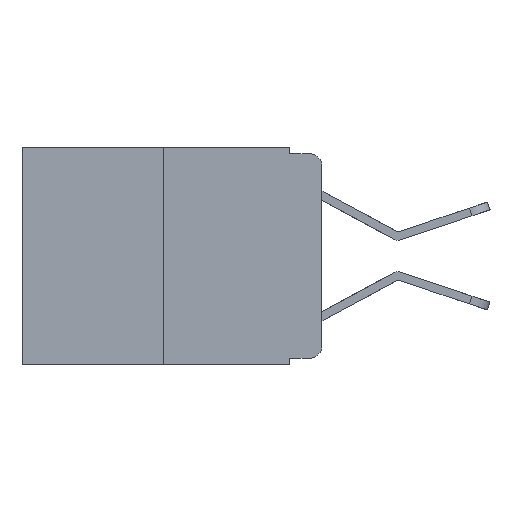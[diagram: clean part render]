
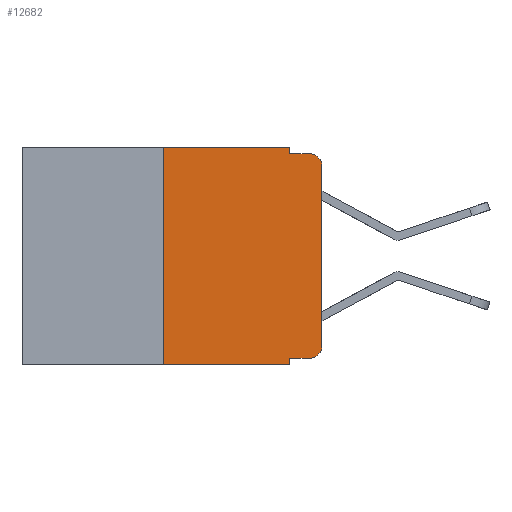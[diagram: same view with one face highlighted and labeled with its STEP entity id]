
A CAD part, left-side view. The second image highlights one B-rep face of the part: STEP entity #12682.
In plain terms, the highlighted planar face has unit normal (-1, 0, 0).
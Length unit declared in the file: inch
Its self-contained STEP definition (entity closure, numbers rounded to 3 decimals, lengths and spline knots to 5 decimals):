
#123 = CIRCLE ( 'NONE', #3753, 0.02 ) ;
#357 = EDGE_CURVE ( 'NONE', #1606, #1124, #11182, .T. ) ;
#536 = DIRECTION ( 'NONE',  ( -1., 0., 0. ) ) ;
#598 = DIRECTION ( 'NONE',  ( 0., 0., -1. ) ) ;
#646 = CARTESIAN_POINT ( 'NONE',  ( 0., 0.473, 0. ) ) ;
#941 = LINE ( 'NONE', #8852, #8374 ) ;
#1074 = VERTEX_POINT ( 'NONE', #6716 ) ;
#1124 = VERTEX_POINT ( 'NONE', #3894 ) ;
#1241 = ORIENTED_EDGE ( 'NONE', *, *, #8033, .F. ) ;
#1576 = VECTOR ( 'NONE', #4683, 39.37008 ) ;
#1606 = VERTEX_POINT ( 'NONE', #9470 ) ;
#1629 = CARTESIAN_POINT ( 'NONE',  ( 0., 0.02, -0.313 ) ) ;
#1958 = CARTESIAN_POINT ( 'NONE',  ( 0., 0., -0.313 ) ) ;
#1969 = AXIS2_PLACEMENT_3D ( 'NONE', #646, #12592, #6759 ) ;
#2442 = EDGE_CURVE ( 'NONE', #8142, #1606, #4233, .T. ) ;
#2474 = CARTESIAN_POINT ( 'NONE',  ( 0., 0.051, 0. ) ) ;
#2570 = LINE ( 'NONE', #2474, #12713 ) ;
#2675 = DIRECTION ( 'NONE',  ( 0., 0., -1. ) ) ;
#2912 = VECTOR ( 'NONE', #5518, 39.37008 ) ;
#3060 = ORIENTED_EDGE ( 'NONE', *, *, #11934, .F. ) ;
#3317 = CARTESIAN_POINT ( 'NONE',  ( 0., 0., 0. ) ) ;
#3336 = DIRECTION ( 'NONE',  ( 0., 0., 1. ) ) ;
#3489 = ORIENTED_EDGE ( 'NONE', *, *, #12116, .T. ) ;
#3708 = ORIENTED_EDGE ( 'NONE', *, *, #10654, .F. ) ;
#3753 = AXIS2_PLACEMENT_3D ( 'NONE', #1629, #8662, #2675 ) ;
#3888 = EDGE_CURVE ( 'NONE', #1074, #8491, #10244, .T. ) ;
#3894 = CARTESIAN_POINT ( 'NONE',  ( 0., 0.02, -0.01 ) ) ;
#4017 = ORIENTED_EDGE ( 'NONE', *, *, #3888, .F. ) ;
#4141 = CARTESIAN_POINT ( 'NONE',  ( 0., 0.25, -0.343 ) ) ;
#4151 = FACE_OUTER_BOUND ( 'NONE', #4937, .T. ) ;
#4233 = LINE ( 'NONE', #3317, #9202 ) ;
#4242 = VERTEX_POINT ( 'NONE', #4947 ) ;
#4360 = VECTOR ( 'NONE', #598, 39.37008 ) ;
#4644 = ORIENTED_EDGE ( 'NONE', *, *, #9358, .F. ) ;
#4681 = CARTESIAN_POINT ( 'NONE',  ( 0., 0.02, -0.03 ) ) ;
#4683 = DIRECTION ( 'NONE',  ( 0., -1., 0. ) ) ;
#4727 = VECTOR ( 'NONE', #10646, 39.37008 ) ;
#4937 = EDGE_LOOP ( 'NONE', ( #10043, #10350, #3060, #3708, #4017, #4644, #3489, #1241, #11802, #7237 ) ) ;
#4947 = CARTESIAN_POINT ( 'NONE',  ( 0., 0.051, -0.333 ) ) ;
#4958 = DIRECTION ( 'NONE',  ( 0., -1., 0. ) ) ;
#5118 = CARTESIAN_POINT ( 'NONE',  ( 0., 0.473, 0. ) ) ;
#5485 = AXIS2_PLACEMENT_3D ( 'NONE', #4681, #536, #12876 ) ;
#5518 = DIRECTION ( 'NONE',  ( 0., -1., 0. ) ) ;
#5755 = PLANE ( 'NONE',  #1969 ) ;
#5876 = LINE ( 'NONE', #10476, #2912 ) ;
#6301 = VERTEX_POINT ( 'NONE', #4141 ) ;
#6519 = CARTESIAN_POINT ( 'NONE',  ( 0., 0.051, 0. ) ) ;
#6714 = EDGE_CURVE ( 'NONE', #7955, #8142, #123, .T. ) ;
#6716 = CARTESIAN_POINT ( 'NONE',  ( 0., 0.25, 0. ) ) ;
#6759 = DIRECTION ( 'NONE',  ( 0., 0., -1. ) ) ;
#6899 = DIRECTION ( 'NONE',  ( 0., -1., 0. ) ) ;
#6993 = LINE ( 'NONE', #11552, #4360 ) ;
#7237 = ORIENTED_EDGE ( 'NONE', *, *, #6714, .T. ) ;
#7372 = EDGE_CURVE ( 'NONE', #4242, #7955, #12125, .T. ) ;
#7450 = DIRECTION ( 'NONE',  ( 0., 0., -1. ) ) ;
#7955 = VERTEX_POINT ( 'NONE', #11296 ) ;
#8033 = EDGE_CURVE ( 'NONE', #4242, #11865, #2570, .T. ) ;
#8142 = VERTEX_POINT ( 'NONE', #1958 ) ;
#8174 = VERTEX_POINT ( 'NONE', #11883 ) ;
#8374 = VECTOR ( 'NONE', #6899, 39.37008 ) ;
#8491 = VERTEX_POINT ( 'NONE', #6519 ) ;
#8605 = CARTESIAN_POINT ( 'NONE',  ( 0., 0.051, -0.333 ) ) ;
#8662 = DIRECTION ( 'NONE',  ( -1., 0., 0. ) ) ;
#8852 = CARTESIAN_POINT ( 'NONE',  ( 0., 0.473, -0.343 ) ) ;
#9202 = VECTOR ( 'NONE', #3336, 39.37008 ) ;
#9358 = EDGE_CURVE ( 'NONE', #6301, #1074, #9681, .T. ) ;
#9367 = CARTESIAN_POINT ( 'NONE',  ( 0., 0.051, -0.343 ) ) ;
#9470 = CARTESIAN_POINT ( 'NONE',  ( 0., 0., -0.03 ) ) ;
#9681 = LINE ( 'NONE', #12572, #4727 ) ;
#10043 = ORIENTED_EDGE ( 'NONE', *, *, #2442, .T. ) ;
#10244 = LINE ( 'NONE', #5118, #12508 ) ;
#10350 = ORIENTED_EDGE ( 'NONE', *, *, #357, .T. ) ;
#10476 = CARTESIAN_POINT ( 'NONE',  ( 0., 0.051, -0.01 ) ) ;
#10646 = DIRECTION ( 'NONE',  ( 0., 0., 1. ) ) ;
#10654 = EDGE_CURVE ( 'NONE', #8491, #8174, #6993, .T. ) ;
#11182 = CIRCLE ( 'NONE', #5485, 0.02 ) ;
#11296 = CARTESIAN_POINT ( 'NONE',  ( 0., 0.02, -0.333 ) ) ;
#11552 = CARTESIAN_POINT ( 'NONE',  ( 0., 0.051, 0. ) ) ;
#11802 = ORIENTED_EDGE ( 'NONE', *, *, #7372, .T. ) ;
#11865 = VERTEX_POINT ( 'NONE', #9367 ) ;
#11883 = CARTESIAN_POINT ( 'NONE',  ( 0., 0.051, -0.01 ) ) ;
#11934 = EDGE_CURVE ( 'NONE', #8174, #1124, #5876, .T. ) ;
#12116 = EDGE_CURVE ( 'NONE', #6301, #11865, #941, .T. ) ;
#12125 = LINE ( 'NONE', #8605, #1576 ) ;
#12508 = VECTOR ( 'NONE', #4958, 39.37008 ) ;
#12572 = CARTESIAN_POINT ( 'NONE',  ( 0., 0.25, 0. ) ) ;
#12592 = DIRECTION ( 'NONE',  ( 1., 0., 0. ) ) ;
#12682 = ADVANCED_FACE ( 'NONE', ( #4151 ), #5755, .F. ) ;
#12713 = VECTOR ( 'NONE', #7450, 39.37008 ) ;
#12876 = DIRECTION ( 'NONE',  ( 0., 0., -1. ) ) ;
